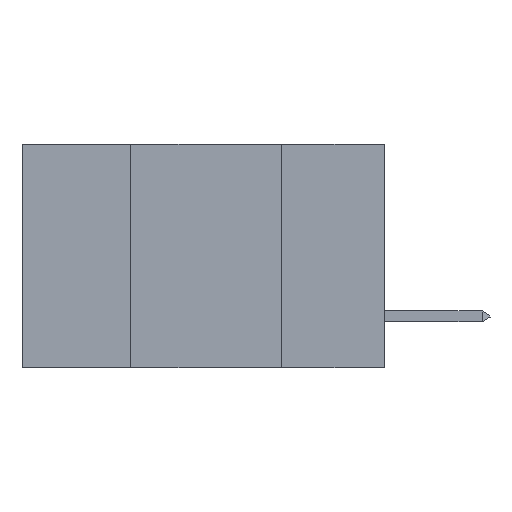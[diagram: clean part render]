
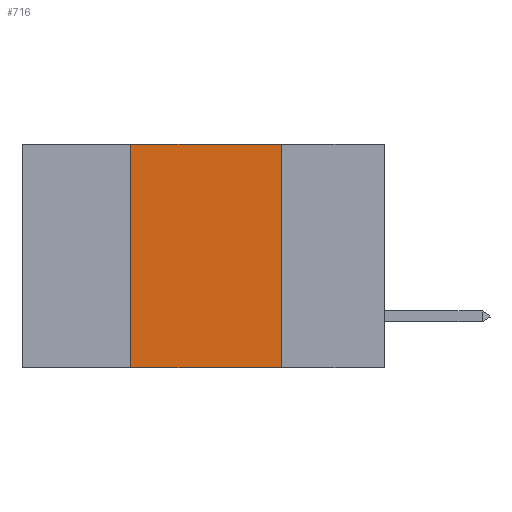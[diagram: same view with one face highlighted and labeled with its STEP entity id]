
A CAD part, left-side view. The second image highlights one B-rep face of the part: STEP entity #716.
In plain terms, the highlighted planar face has unit normal (-1, 0, 0).
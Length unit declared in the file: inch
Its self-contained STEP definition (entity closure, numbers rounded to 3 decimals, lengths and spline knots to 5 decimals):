
#156 = CARTESIAN_POINT ( 'NONE',  ( 0., 0.42, 0. ) ) ;
#716 = ADVANCED_FACE ( 'NONE', ( #8786 ), #12474, .F. ) ;
#857 = CARTESIAN_POINT ( 'NONE',  ( 0., 0.42, 0. ) ) ;
#989 = VERTEX_POINT ( 'NONE', #156 ) ;
#2234 = CARTESIAN_POINT ( 'NONE',  ( 0., 0.6, 0. ) ) ;
#3009 = LINE ( 'NONE', #13799, #18040 ) ;
#4428 = VERTEX_POINT ( 'NONE', #12852 ) ;
#4820 = CARTESIAN_POINT ( 'NONE',  ( 0., 0.6, 0. ) ) ;
#4860 = CARTESIAN_POINT ( 'NONE',  ( 0., 0.17, 0. ) ) ;
#5411 = DIRECTION ( 'NONE',  ( 0., 0., -1. ) ) ;
#5660 = LINE ( 'NONE', #14606, #6590 ) ;
#5724 = VERTEX_POINT ( 'NONE', #4860 ) ;
#6188 = VERTEX_POINT ( 'NONE', #15787 ) ;
#6385 = DIRECTION ( 'NONE',  ( 0., 0., -1. ) ) ;
#6590 = VECTOR ( 'NONE', #10328, 39.37008 ) ;
#8786 = FACE_OUTER_BOUND ( 'NONE', #13724, .T. ) ;
#9448 = DIRECTION ( 'NONE',  ( 0., 0., 1. ) ) ;
#10328 = DIRECTION ( 'NONE',  ( 0., -1., 0. ) ) ;
#10568 = EDGE_CURVE ( 'NONE', #4428, #989, #10769, .T. ) ;
#10769 = LINE ( 'NONE', #857, #11931 ) ;
#11013 = DIRECTION ( 'NONE',  ( 1., 0., 0. ) ) ;
#11346 = EDGE_CURVE ( 'NONE', #5724, #6188, #3009, .T. ) ;
#11618 = AXIS2_PLACEMENT_3D ( 'NONE', #2234, #11013, #5411 ) ;
#11931 = VECTOR ( 'NONE', #9448, 39.37008 ) ;
#12218 = VECTOR ( 'NONE', #17925, 39.37008 ) ;
#12474 = PLANE ( 'NONE',  #11618 ) ;
#12852 = CARTESIAN_POINT ( 'NONE',  ( 0., 0.42, -0.37 ) ) ;
#13282 = EDGE_CURVE ( 'NONE', #4428, #6188, #5660, .T. ) ;
#13724 = EDGE_LOOP ( 'NONE', ( #16584, #14753, #14990, #17724 ) ) ;
#13799 = CARTESIAN_POINT ( 'NONE',  ( 0., 0.17, 0. ) ) ;
#14529 = LINE ( 'NONE', #4820, #12218 ) ;
#14606 = CARTESIAN_POINT ( 'NONE',  ( 0., 0.6, -0.37 ) ) ;
#14753 = ORIENTED_EDGE ( 'NONE', *, *, #14845, .F. ) ;
#14845 = EDGE_CURVE ( 'NONE', #989, #5724, #14529, .T. ) ;
#14990 = ORIENTED_EDGE ( 'NONE', *, *, #10568, .F. ) ;
#15787 = CARTESIAN_POINT ( 'NONE',  ( 0., 0.17, -0.37 ) ) ;
#16584 = ORIENTED_EDGE ( 'NONE', *, *, #11346, .F. ) ;
#17724 = ORIENTED_EDGE ( 'NONE', *, *, #13282, .T. ) ;
#17925 = DIRECTION ( 'NONE',  ( 0., -1., 0. ) ) ;
#18040 = VECTOR ( 'NONE', #6385, 39.37008 ) ;
